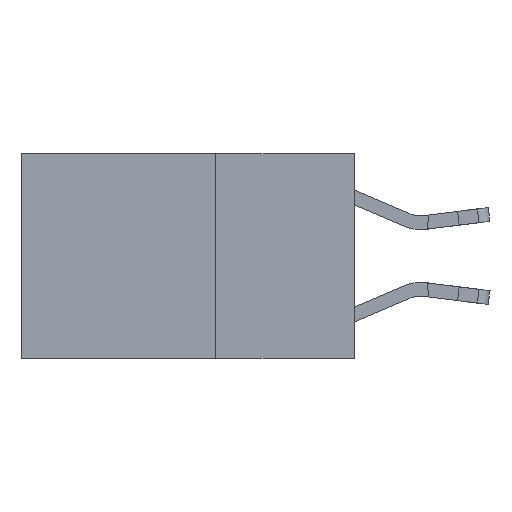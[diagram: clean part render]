
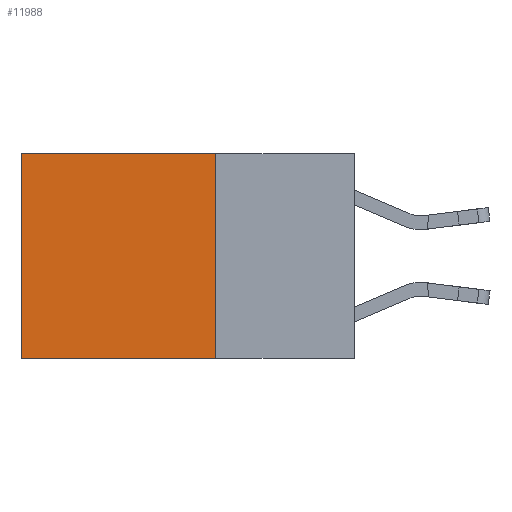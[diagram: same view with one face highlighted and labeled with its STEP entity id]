
A CAD part, left-side view. The second image highlights one B-rep face of the part: STEP entity #11988.
In plain terms, the highlighted planar face has unit normal (-1, 0, 0).
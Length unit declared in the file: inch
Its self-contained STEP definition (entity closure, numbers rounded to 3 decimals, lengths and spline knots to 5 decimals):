
#82 = DIRECTION ( 'NONE',  ( 0., 0., -1. ) ) ;
#1185 = EDGE_CURVE ( 'NONE', #7284, #2771, #5752, .T. ) ;
#1691 = EDGE_CURVE ( 'NONE', #2771, #3616, #11169, .T. ) ;
#2320 = DIRECTION ( 'NONE',  ( 0., 0., -1. ) ) ;
#2432 = ORIENTED_EDGE ( 'NONE', *, *, #9142, .T. ) ;
#2525 = VECTOR ( 'NONE', #5118, 39.37008 ) ;
#2561 = CARTESIAN_POINT ( 'NONE',  ( 0.2625, 0.6, 0. ) ) ;
#2592 = ORIENTED_EDGE ( 'NONE', *, *, #1185, .F. ) ;
#2606 = CARTESIAN_POINT ( 'NONE',  ( 0.2625, 0.25, -0.37 ) ) ;
#2756 = VECTOR ( 'NONE', #2320, 39.37008 ) ;
#2771 = VERTEX_POINT ( 'NONE', #2606 ) ;
#3030 = VECTOR ( 'NONE', #6103, 39.37008 ) ;
#3616 = VERTEX_POINT ( 'NONE', #6914 ) ;
#3734 = ORIENTED_EDGE ( 'NONE', *, *, #11241, .T. ) ;
#4128 = FACE_OUTER_BOUND ( 'NONE', #8211, .T. ) ;
#5118 = DIRECTION ( 'NONE',  ( 0., 1., 0. ) ) ;
#5752 = LINE ( 'NONE', #8935, #3030 ) ;
#6103 = DIRECTION ( 'NONE',  ( 0., 0., -1. ) ) ;
#6251 = DIRECTION ( 'NONE',  ( 1., 0., 0. ) ) ;
#6514 = AXIS2_PLACEMENT_3D ( 'NONE', #12361, #6251, #82 ) ;
#6820 = ORIENTED_EDGE ( 'NONE', *, *, #1691, .F. ) ;
#6914 = CARTESIAN_POINT ( 'NONE',  ( 0.2625, 0.6, -0.37 ) ) ;
#7044 = VERTEX_POINT ( 'NONE', #2561 ) ;
#7284 = VERTEX_POINT ( 'NONE', #12137 ) ;
#7925 = DIRECTION ( 'NONE',  ( 0., 1., 0. ) ) ;
#7977 = LINE ( 'NONE', #12255, #2525 ) ;
#8211 = EDGE_LOOP ( 'NONE', ( #2432, #6820, #2592, #3734 ) ) ;
#8935 = CARTESIAN_POINT ( 'NONE',  ( 0.2625, 0.25, 0. ) ) ;
#8980 = CARTESIAN_POINT ( 'NONE',  ( 0.2625, 0.25, -0.37 ) ) ;
#9142 = EDGE_CURVE ( 'NONE', #7044, #3616, #10904, .T. ) ;
#9281 = PLANE ( 'NONE',  #6514 ) ;
#10904 = LINE ( 'NONE', #11522, #2756 ) ;
#11169 = LINE ( 'NONE', #8980, #13213 ) ;
#11241 = EDGE_CURVE ( 'NONE', #7284, #7044, #7977, .T. ) ;
#11522 = CARTESIAN_POINT ( 'NONE',  ( 0.2625, 0.6, 0. ) ) ;
#11988 = ADVANCED_FACE ( 'NONE', ( #4128 ), #9281, .F. ) ;
#12137 = CARTESIAN_POINT ( 'NONE',  ( 0.2625, 0.25, 0. ) ) ;
#12255 = CARTESIAN_POINT ( 'NONE',  ( 0.2625, 0.25, 0. ) ) ;
#12361 = CARTESIAN_POINT ( 'NONE',  ( 0.2625, 0.25, 0. ) ) ;
#13213 = VECTOR ( 'NONE', #7925, 39.37008 ) ;
